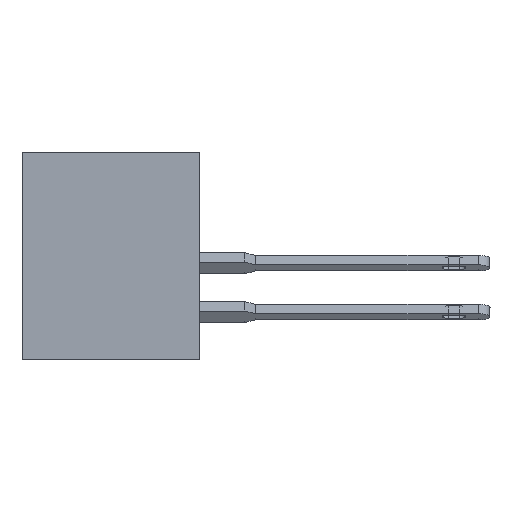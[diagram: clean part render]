
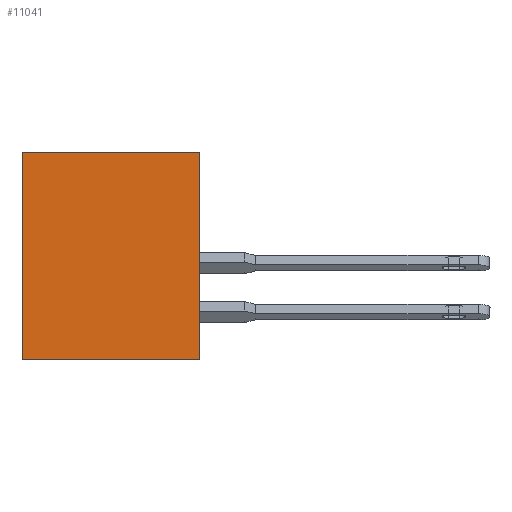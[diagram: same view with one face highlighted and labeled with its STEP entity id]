
A CAD part, left-side view. The second image highlights one B-rep face of the part: STEP entity #11041.
In plain terms, the highlighted planar face has unit normal (-1, 0, 0).
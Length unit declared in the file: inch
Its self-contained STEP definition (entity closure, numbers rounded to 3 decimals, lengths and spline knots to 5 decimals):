
#3 = ORIENTED_EDGE ( 'NONE', *, *, #23777, .T. ) ;
#1656 = DIRECTION ( 'NONE',  ( 0., -1., 0. ) ) ;
#2603 = ORIENTED_EDGE ( 'NONE', *, *, #23808, .T. ) ;
#3450 = CARTESIAN_POINT ( 'NONE',  ( 0., 0., 0. ) ) ;
#3557 = PLANE ( 'NONE',  #24210 ) ;
#4163 = DIRECTION ( 'NONE',  ( 0., -1., 0. ) ) ;
#5435 = VERTEX_POINT ( 'NONE', #25542 ) ;
#6581 = VECTOR ( 'NONE', #20897, 39.37008 ) ;
#7064 = FACE_OUTER_BOUND ( 'NONE', #13899, .T. ) ;
#7075 = LINE ( 'NONE', #19877, #23700 ) ;
#7534 = VECTOR ( 'NONE', #4163, 39.37008 ) ;
#9052 = CARTESIAN_POINT ( 'NONE',  ( 0., 0., -0.531 ) ) ;
#10017 = CARTESIAN_POINT ( 'NONE',  ( 0., 0., 0. ) ) ;
#10727 = CARTESIAN_POINT ( 'NONE',  ( 0., 0.453, 0. ) ) ;
#10809 = VERTEX_POINT ( 'NONE', #9052 ) ;
#11041 = ADVANCED_FACE ( 'NONE', ( #7064 ), #3557, .F. ) ;
#11604 = VERTEX_POINT ( 'NONE', #18441 ) ;
#12077 = CARTESIAN_POINT ( 'NONE',  ( 0., 0.453, 0. ) ) ;
#13899 = EDGE_LOOP ( 'NONE', ( #3, #23785, #24396, #2603 ) ) ;
#16386 = DIRECTION ( 'NONE',  ( 1., 0., 0. ) ) ;
#16613 = EDGE_CURVE ( 'NONE', #11604, #26305, #23511, .T. ) ;
#18441 = CARTESIAN_POINT ( 'NONE',  ( 0., 0.453, 0. ) ) ;
#19877 = CARTESIAN_POINT ( 'NONE',  ( 0., 0.453, 0. ) ) ;
#19960 = DIRECTION ( 'NONE',  ( 0., 0., 1. ) ) ;
#20897 = DIRECTION ( 'NONE',  ( 0., 0., 1. ) ) ;
#21556 = VECTOR ( 'NONE', #1656, 39.37008 ) ;
#23511 = LINE ( 'NONE', #10727, #7534 ) ;
#23700 = VECTOR ( 'NONE', #19960, 39.37008 ) ;
#23777 = EDGE_CURVE ( 'NONE', #10809, #26305, #25206, .T. ) ;
#23785 = ORIENTED_EDGE ( 'NONE', *, *, #16613, .F. ) ;
#23808 = EDGE_CURVE ( 'NONE', #5435, #10809, #26228, .T. ) ;
#24210 = AXIS2_PLACEMENT_3D ( 'NONE', #12077, #16386, #27002 ) ;
#24396 = ORIENTED_EDGE ( 'NONE', *, *, #26741, .F. ) ;
#25187 = CARTESIAN_POINT ( 'NONE',  ( 0., 0.453, -0.531 ) ) ;
#25206 = LINE ( 'NONE', #10017, #6581 ) ;
#25542 = CARTESIAN_POINT ( 'NONE',  ( 0., 0.453, -0.531 ) ) ;
#26228 = LINE ( 'NONE', #25187, #21556 ) ;
#26305 = VERTEX_POINT ( 'NONE', #3450 ) ;
#26741 = EDGE_CURVE ( 'NONE', #5435, #11604, #7075, .T. ) ;
#27002 = DIRECTION ( 'NONE',  ( 0., 0., -1. ) ) ;
